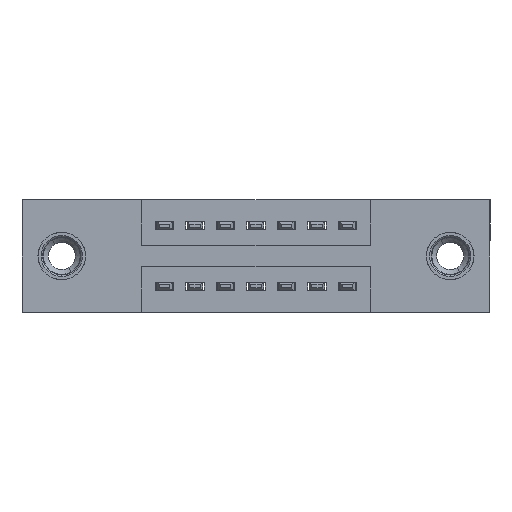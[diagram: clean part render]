
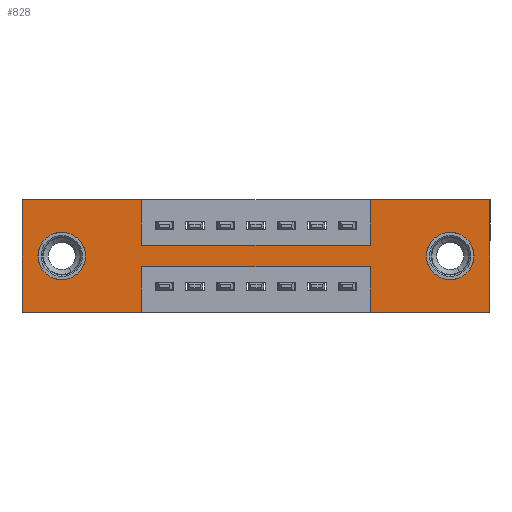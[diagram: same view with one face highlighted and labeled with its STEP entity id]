
A CAD part, front view. The second image highlights one B-rep face of the part: STEP entity #828.
In plain terms, the highlighted planar face has unit normal (0, -1, 0).
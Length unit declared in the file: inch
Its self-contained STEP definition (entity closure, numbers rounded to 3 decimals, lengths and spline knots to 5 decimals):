
#329 = LINE ( 'NONE', #690, #14069 ) ;
#340 = LINE ( 'NONE', #818, #6928 ) ;
#419 = CARTESIAN_POINT ( 'NONE',  ( 1.405, 0., -0.107 ) ) ;
#441 = EDGE_CURVE ( 'NONE', #10674, #12754, #12433, .T. ) ;
#494 = LINE ( 'NONE', #3273, #1017 ) ;
#506 = ORIENTED_EDGE ( 'NONE', *, *, #3031, .F. ) ;
#513 = DIRECTION ( 'NONE',  ( 0., 1., 0. ) ) ;
#647 = CARTESIAN_POINT ( 'NONE',  ( 0.13, 0., -0.263 ) ) ;
#690 = CARTESIAN_POINT ( 'NONE',  ( 1.1425, 0., 0. ) ) ;
#757 = CIRCLE ( 'NONE', #8964, 0.078 ) ;
#791 = DIRECTION ( 'NONE',  ( -1., 0., 0. ) ) ;
#818 = CARTESIAN_POINT ( 'NONE',  ( 0., 0., 0. ) ) ;
#828 = ADVANCED_FACE ( 'NONE', ( #10253, #8265, #3843 ), #2286, .T. ) ;
#1017 = VECTOR ( 'NONE', #6751, 39.37008 ) ;
#1145 = CARTESIAN_POINT ( 'NONE',  ( 0.13, 0., -0.185 ) ) ;
#1195 = DIRECTION ( 'NONE',  ( 0., 1., 0. ) ) ;
#1431 = CARTESIAN_POINT ( 'NONE',  ( 0.3925, 0., -0.37 ) ) ;
#1527 = VECTOR ( 'NONE', #791, 39.37008 ) ;
#1716 = ORIENTED_EDGE ( 'NONE', *, *, #6237, .F. ) ;
#1729 = VERTEX_POINT ( 'NONE', #419 ) ;
#1822 = CARTESIAN_POINT ( 'NONE',  ( 1.405, 0., -0.185 ) ) ;
#1879 = CARTESIAN_POINT ( 'NONE',  ( 0.3925, 0., 0. ) ) ;
#2039 = EDGE_CURVE ( 'NONE', #12754, #13338, #494, .T. ) ;
#2081 = CARTESIAN_POINT ( 'NONE',  ( 1.535, 0., 0. ) ) ;
#2286 = PLANE ( 'NONE',  #4657 ) ;
#2930 = VECTOR ( 'NONE', #8829, 39.37008 ) ;
#2954 = DIRECTION ( 'NONE',  ( 0., 0., 1. ) ) ;
#3031 = EDGE_CURVE ( 'NONE', #6818, #11411, #8288, .T. ) ;
#3053 = ORIENTED_EDGE ( 'NONE', *, *, #7603, .T. ) ;
#3092 = DIRECTION ( 'NONE',  ( 1., 0., 0. ) ) ;
#3144 = CARTESIAN_POINT ( 'NONE',  ( 0.13, 0., -0.107 ) ) ;
#3250 = ORIENTED_EDGE ( 'NONE', *, *, #13406, .F. ) ;
#3272 = DIRECTION ( 'NONE',  ( 0., 0., 1. ) ) ;
#3273 = CARTESIAN_POINT ( 'NONE',  ( 0., 0., -0.37 ) ) ;
#3309 = DIRECTION ( 'NONE',  ( 0., 1., 0. ) ) ;
#3539 = CARTESIAN_POINT ( 'NONE',  ( 1.1425, 0., -0.37 ) ) ;
#3666 = EDGE_LOOP ( 'NONE', ( #6123, #9504, #1716, #13796, #5749, #3250, #14632, #9793, #506, #7227, #6351, #14797 ) ) ;
#3763 = ORIENTED_EDGE ( 'NONE', *, *, #10493, .T. ) ;
#3843 = FACE_OUTER_BOUND ( 'NONE', #3666, .T. ) ;
#4121 = CARTESIAN_POINT ( 'NONE',  ( 1.535, 0., -0.37 ) ) ;
#4126 = DIRECTION ( 'NONE',  ( 0., 0., -1. ) ) ;
#4387 = CARTESIAN_POINT ( 'NONE',  ( 0.3925, 0., -0.22 ) ) ;
#4499 = VECTOR ( 'NONE', #14284, 39.37008 ) ;
#4559 = CARTESIAN_POINT ( 'NONE',  ( 0., 0., 0. ) ) ;
#4657 = AXIS2_PLACEMENT_3D ( 'NONE', #10301, #11318, #10217 ) ;
#4742 = CARTESIAN_POINT ( 'NONE',  ( 1.1425, 0., 0. ) ) ;
#4941 = LINE ( 'NONE', #1431, #6356 ) ;
#4944 = LINE ( 'NONE', #14184, #1527 ) ;
#4971 = LINE ( 'NONE', #14319, #9552 ) ;
#5054 = EDGE_LOOP ( 'NONE', ( #8434, #8845 ) ) ;
#5105 = DIRECTION ( 'NONE',  ( 0., 0., -1. ) ) ;
#5135 = VERTEX_POINT ( 'NONE', #4742 ) ;
#5283 = EDGE_CURVE ( 'NONE', #9118, #6474, #14334, .T. ) ;
#5401 = VERTEX_POINT ( 'NONE', #5416 ) ;
#5416 = CARTESIAN_POINT ( 'NONE',  ( 1.1425, 0., -0.22 ) ) ;
#5471 = DIRECTION ( 'NONE',  ( 0., 0., -1. ) ) ;
#5749 = ORIENTED_EDGE ( 'NONE', *, *, #441, .F. ) ;
#5783 = LINE ( 'NONE', #3539, #11103 ) ;
#5943 = CIRCLE ( 'NONE', #8212, 0.078 ) ;
#6123 = ORIENTED_EDGE ( 'NONE', *, *, #11470, .F. ) ;
#6202 = DIRECTION ( 'NONE',  ( 0., 1., 0. ) ) ;
#6237 = EDGE_CURVE ( 'NONE', #13338, #5401, #5783, .T. ) ;
#6303 = DIRECTION ( 'NONE',  ( 0., 0., -1. ) ) ;
#6351 = ORIENTED_EDGE ( 'NONE', *, *, #10558, .F. ) ;
#6356 = VECTOR ( 'NONE', #5105, 39.37008 ) ;
#6474 = VERTEX_POINT ( 'NONE', #647 ) ;
#6670 = CARTESIAN_POINT ( 'NONE',  ( 1.1425, 0., -0.37 ) ) ;
#6751 = DIRECTION ( 'NONE',  ( -1., 0., 0. ) ) ;
#6818 = VERTEX_POINT ( 'NONE', #11293 ) ;
#6928 = VECTOR ( 'NONE', #3092, 39.37008 ) ;
#7200 = CARTESIAN_POINT ( 'NONE',  ( 0.3925, 0., -0.15 ) ) ;
#7227 = ORIENTED_EDGE ( 'NONE', *, *, #9133, .F. ) ;
#7444 = LINE ( 'NONE', #9675, #4499 ) ;
#7454 = CARTESIAN_POINT ( 'NONE',  ( 1.405, 0., -0.263 ) ) ;
#7603 = EDGE_CURVE ( 'NONE', #1729, #9531, #757, .T. ) ;
#7648 = CARTESIAN_POINT ( 'NONE',  ( 1.405, 0., -0.185 ) ) ;
#7685 = CARTESIAN_POINT ( 'NONE',  ( 0., 0., 0. ) ) ;
#7990 = CARTESIAN_POINT ( 'NONE',  ( 0.3925, 0., -0.37 ) ) ;
#8048 = VERTEX_POINT ( 'NONE', #10635 ) ;
#8212 = AXIS2_PLACEMENT_3D ( 'NONE', #9628, #513, #8473 ) ;
#8265 = FACE_BOUND ( 'NONE', #5054, .T. ) ;
#8288 = LINE ( 'NONE', #1879, #11358 ) ;
#8382 = VECTOR ( 'NONE', #6303, 39.37008 ) ;
#8434 = ORIENTED_EDGE ( 'NONE', *, *, #5283, .T. ) ;
#8473 = DIRECTION ( 'NONE',  ( 0., 0., 1. ) ) ;
#8654 = EDGE_CURVE ( 'NONE', #11411, #8048, #7444, .T. ) ;
#8719 = DIRECTION ( 'NONE',  ( 0., 0., 1. ) ) ;
#8829 = DIRECTION ( 'NONE',  ( 1., 0., 0. ) ) ;
#8840 = CIRCLE ( 'NONE', #10812, 0.078 ) ;
#8845 = ORIENTED_EDGE ( 'NONE', *, *, #14471, .T. ) ;
#8964 = AXIS2_PLACEMENT_3D ( 'NONE', #7648, #3309, #5471 ) ;
#9118 = VERTEX_POINT ( 'NONE', #3144 ) ;
#9133 = EDGE_CURVE ( 'NONE', #9220, #6818, #340, .T. ) ;
#9209 = AXIS2_PLACEMENT_3D ( 'NONE', #1145, #1195, #3272 ) ;
#9220 = VERTEX_POINT ( 'NONE', #4559 ) ;
#9504 = ORIENTED_EDGE ( 'NONE', *, *, #11997, .F. ) ;
#9531 = VERTEX_POINT ( 'NONE', #7454 ) ;
#9545 = EDGE_CURVE ( 'NONE', #8048, #5135, #329, .T. ) ;
#9552 = VECTOR ( 'NONE', #2954, 39.37008 ) ;
#9628 = CARTESIAN_POINT ( 'NONE',  ( 0.13, 0., -0.185 ) ) ;
#9675 = CARTESIAN_POINT ( 'NONE',  ( 0.3925, 0., -0.15 ) ) ;
#9734 = LINE ( 'NONE', #10129, #12438 ) ;
#9793 = ORIENTED_EDGE ( 'NONE', *, *, #8654, .F. ) ;
#9930 = VERTEX_POINT ( 'NONE', #7990 ) ;
#10129 = CARTESIAN_POINT ( 'NONE',  ( 0., 0., -0.37 ) ) ;
#10217 = DIRECTION ( 'NONE',  ( 0., 0., -1. ) ) ;
#10253 = FACE_BOUND ( 'NONE', #11551, .T. ) ;
#10301 = CARTESIAN_POINT ( 'NONE',  ( 0., 0., -0.37 ) ) ;
#10493 = EDGE_CURVE ( 'NONE', #9531, #1729, #8840, .T. ) ;
#10558 = EDGE_CURVE ( 'NONE', #13646, #9220, #4971, .T. ) ;
#10635 = CARTESIAN_POINT ( 'NONE',  ( 1.1425, 0., -0.15 ) ) ;
#10674 = VERTEX_POINT ( 'NONE', #2081 ) ;
#10787 = EDGE_CURVE ( 'NONE', #9930, #13646, #9734, .T. ) ;
#10812 = AXIS2_PLACEMENT_3D ( 'NONE', #1822, #6202, #14175 ) ;
#10965 = CARTESIAN_POINT ( 'NONE',  ( 1.535, 0., 0. ) ) ;
#11103 = VECTOR ( 'NONE', #13799, 39.37008 ) ;
#11256 = DIRECTION ( 'NONE',  ( -1., 0., 0. ) ) ;
#11293 = CARTESIAN_POINT ( 'NONE',  ( 0.3925, 0., 0. ) ) ;
#11318 = DIRECTION ( 'NONE',  ( 0., -1., 0. ) ) ;
#11358 = VECTOR ( 'NONE', #4126, 39.37008 ) ;
#11411 = VERTEX_POINT ( 'NONE', #7200 ) ;
#11470 = EDGE_CURVE ( 'NONE', #14051, #9930, #4941, .T. ) ;
#11551 = EDGE_LOOP ( 'NONE', ( #3053, #3763 ) ) ;
#11997 = EDGE_CURVE ( 'NONE', #5401, #14051, #4944, .T. ) ;
#12433 = LINE ( 'NONE', #10965, #8382 ) ;
#12438 = VECTOR ( 'NONE', #11256, 39.37008 ) ;
#12754 = VERTEX_POINT ( 'NONE', #4121 ) ;
#13338 = VERTEX_POINT ( 'NONE', #6670 ) ;
#13406 = EDGE_CURVE ( 'NONE', #5135, #10674, #13816, .T. ) ;
#13646 = VERTEX_POINT ( 'NONE', #14675 ) ;
#13796 = ORIENTED_EDGE ( 'NONE', *, *, #2039, .F. ) ;
#13799 = DIRECTION ( 'NONE',  ( 0., 0., 1. ) ) ;
#13816 = LINE ( 'NONE', #7685, #2930 ) ;
#14051 = VERTEX_POINT ( 'NONE', #4387 ) ;
#14069 = VECTOR ( 'NONE', #8719, 39.37008 ) ;
#14175 = DIRECTION ( 'NONE',  ( 0., 0., -1. ) ) ;
#14184 = CARTESIAN_POINT ( 'NONE',  ( 0.3925, 0., -0.22 ) ) ;
#14284 = DIRECTION ( 'NONE',  ( 1., 0., 0. ) ) ;
#14319 = CARTESIAN_POINT ( 'NONE',  ( 0., 0., 0. ) ) ;
#14334 = CIRCLE ( 'NONE', #9209, 0.078 ) ;
#14471 = EDGE_CURVE ( 'NONE', #6474, #9118, #5943, .T. ) ;
#14632 = ORIENTED_EDGE ( 'NONE', *, *, #9545, .F. ) ;
#14675 = CARTESIAN_POINT ( 'NONE',  ( 0., 0., -0.37 ) ) ;
#14797 = ORIENTED_EDGE ( 'NONE', *, *, #10787, .F. ) ;
